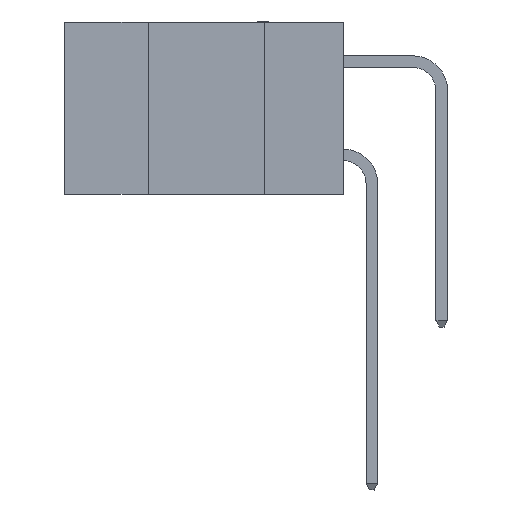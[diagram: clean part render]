
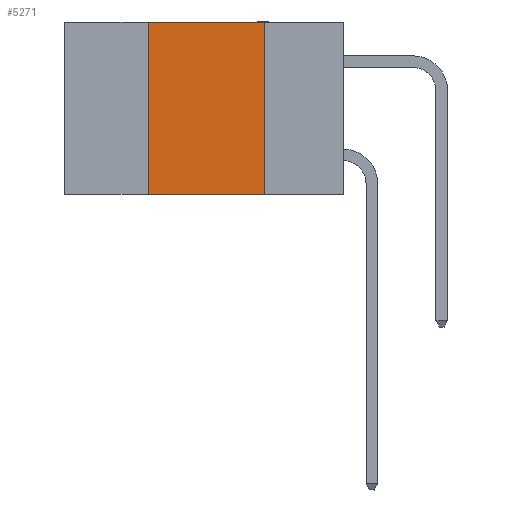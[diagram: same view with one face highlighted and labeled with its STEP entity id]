
A CAD part, left-side view. The second image highlights one B-rep face of the part: STEP entity #5271.
In plain terms, the highlighted planar face has unit normal (-1, 0, 0).
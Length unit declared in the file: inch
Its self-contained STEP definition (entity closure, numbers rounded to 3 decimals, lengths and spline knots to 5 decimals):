
#1650 = VERTEX_POINT ( 'NONE', #3866 ) ;
#1781 = EDGE_CURVE ( 'NONE', #13198, #20786, #4751, .T. ) ;
#2591 = EDGE_CURVE ( 'NONE', #22182, #1650, #11444, .T. ) ;
#3866 = CARTESIAN_POINT ( 'NONE',  ( 0., 0.17, 0. ) ) ;
#4751 = LINE ( 'NONE', #31847, #32750 ) ;
#4971 = AXIS2_PLACEMENT_3D ( 'NONE', #17835, #28649, #14751 ) ;
#5120 = VECTOR ( 'NONE', #24627, 39.37008 ) ;
#5158 = LINE ( 'NONE', #34379, #26785 ) ;
#5271 = ADVANCED_FACE ( 'NONE', ( #27346 ), #14874, .F. ) ;
#6537 = LINE ( 'NONE', #21484, #6991 ) ;
#6901 = ORIENTED_EDGE ( 'NONE', *, *, #14451, .F. ) ;
#6991 = VECTOR ( 'NONE', #16504, 39.37008 ) ;
#11444 = LINE ( 'NONE', #27825, #5120 ) ;
#13198 = VERTEX_POINT ( 'NONE', #20791 ) ;
#14451 = EDGE_CURVE ( 'NONE', #1650, #20786, #5158, .T. ) ;
#14751 = DIRECTION ( 'NONE',  ( 0., 0., -1. ) ) ;
#14792 = ORIENTED_EDGE ( 'NONE', *, *, #1781, .T. ) ;
#14874 = PLANE ( 'NONE',  #4971 ) ;
#15011 = EDGE_LOOP ( 'NONE', ( #6901, #17169, #25624, #14792 ) ) ;
#16504 = DIRECTION ( 'NONE',  ( 0., 0., 1. ) ) ;
#16932 = CARTESIAN_POINT ( 'NONE',  ( 0., 0.17, -0.37 ) ) ;
#17169 = ORIENTED_EDGE ( 'NONE', *, *, #2591, .F. ) ;
#17835 = CARTESIAN_POINT ( 'NONE',  ( 0., 0.6, 0. ) ) ;
#20786 = VERTEX_POINT ( 'NONE', #16932 ) ;
#20791 = CARTESIAN_POINT ( 'NONE',  ( 0., 0.42, -0.37 ) ) ;
#21484 = CARTESIAN_POINT ( 'NONE',  ( 0., 0.42, 0. ) ) ;
#22182 = VERTEX_POINT ( 'NONE', #31427 ) ;
#22991 = EDGE_CURVE ( 'NONE', #13198, #22182, #6537, .T. ) ;
#23511 = DIRECTION ( 'NONE',  ( 0., -1., 0. ) ) ;
#24627 = DIRECTION ( 'NONE',  ( 0., -1., 0. ) ) ;
#25624 = ORIENTED_EDGE ( 'NONE', *, *, #22991, .F. ) ;
#26785 = VECTOR ( 'NONE', #28932, 39.37008 ) ;
#27346 = FACE_OUTER_BOUND ( 'NONE', #15011, .T. ) ;
#27825 = CARTESIAN_POINT ( 'NONE',  ( 0., 0.6, 0. ) ) ;
#28649 = DIRECTION ( 'NONE',  ( 1., 0., 0. ) ) ;
#28932 = DIRECTION ( 'NONE',  ( 0., 0., -1. ) ) ;
#31427 = CARTESIAN_POINT ( 'NONE',  ( 0., 0.42, 0. ) ) ;
#31847 = CARTESIAN_POINT ( 'NONE',  ( 0., 0.6, -0.37 ) ) ;
#32750 = VECTOR ( 'NONE', #23511, 39.37008 ) ;
#34379 = CARTESIAN_POINT ( 'NONE',  ( 0., 0.17, 0. ) ) ;
